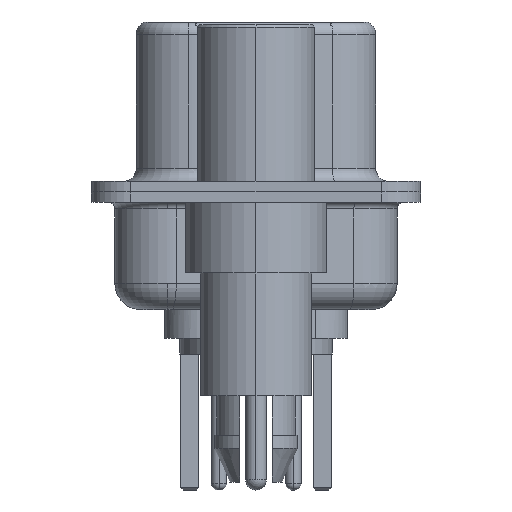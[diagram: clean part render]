
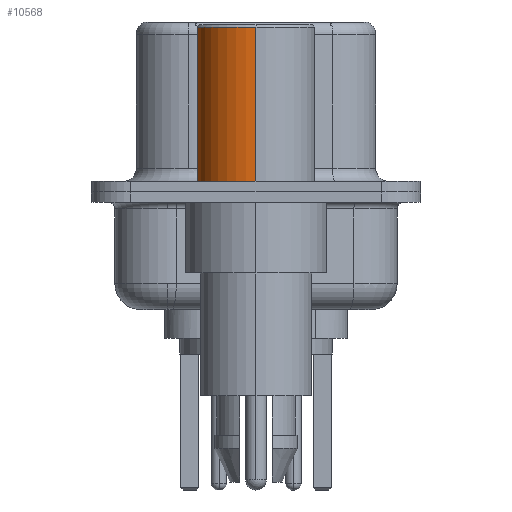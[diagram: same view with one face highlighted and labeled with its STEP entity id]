
A CAD part, left-side view. The second image highlights one B-rep face of the part: STEP entity #10568.
In plain terms, the highlighted cylindrical face has radius 2.25 mm (diameter 4.5 mm), a partial arc.
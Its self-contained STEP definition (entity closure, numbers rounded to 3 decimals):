
#782 = AXIS2_PLACEMENT_3D ( 'NONE', #19846, #8580, #21734 ) ;
#1077 = EDGE_CURVE ( 'NONE', #3015, #3858, #3713, .T. ) ;
#1628 = CYLINDRICAL_SURFACE ( 'NONE', #24458, 2.25 ) ;
#1768 = CARTESIAN_POINT ( 'NONE',  ( 2.25, 0., 0.4 ) ) ;
#3015 = VERTEX_POINT ( 'NONE', #21162 ) ;
#3284 = VERTEX_POINT ( 'NONE', #10674 ) ;
#3713 = CIRCLE ( 'NONE', #12100, 2.25 ) ;
#3714 = VECTOR ( 'NONE', #23561, 1000. ) ;
#3858 = VERTEX_POINT ( 'NONE', #18015 ) ;
#4449 = EDGE_CURVE ( 'NONE', #3284, #3858, #23678, .T. ) ;
#4867 = CARTESIAN_POINT ( 'NONE',  ( 0., 0., 0.581 ) ) ;
#6761 = DIRECTION ( 'NONE',  ( 1., 0., 0. ) ) ;
#6803 = DIRECTION ( 'NONE',  ( 0., 0., 1. ) ) ;
#7287 = FACE_OUTER_BOUND ( 'NONE', #14802, .T. ) ;
#7501 = ORIENTED_EDGE ( 'NONE', *, *, #12702, .F. ) ;
#7556 = CIRCLE ( 'NONE', #782, 2.25 ) ;
#8580 = DIRECTION ( 'NONE',  ( 0., 0., 1. ) ) ;
#8598 = CARTESIAN_POINT ( 'NONE',  ( 0., 0., 6.3 ) ) ;
#8698 = VECTOR ( 'NONE', #17284, 1000. ) ;
#9373 = LINE ( 'NONE', #14204, #3714 ) ;
#10568 = ADVANCED_FACE ( 'NONE', ( #7287 ), #1628, .T. ) ;
#10674 = CARTESIAN_POINT ( 'NONE',  ( -2.25, 0., 0.4 ) ) ;
#10982 = ORIENTED_EDGE ( 'NONE', *, *, #4449, .T. ) ;
#12100 = AXIS2_PLACEMENT_3D ( 'NONE', #8598, #6803, #6761 ) ;
#12702 = EDGE_CURVE ( 'NONE', #19231, #3015, #9373, .T. ) ;
#12870 = ORIENTED_EDGE ( 'NONE', *, *, #1077, .F. ) ;
#13349 = EDGE_CURVE ( 'NONE', #19231, #3284, #7556, .T. ) ;
#13755 = CARTESIAN_POINT ( 'NONE',  ( -2.25, 0., 0.581 ) ) ;
#14204 = CARTESIAN_POINT ( 'NONE',  ( 2.25, 0., 0.581 ) ) ;
#14802 = EDGE_LOOP ( 'NONE', ( #22408, #10982, #12870, #7501 ) ) ;
#16181 = DIRECTION ( 'NONE',  ( 0., 0., 1. ) ) ;
#17284 = DIRECTION ( 'NONE',  ( 0., 0., 1. ) ) ;
#17964 = DIRECTION ( 'NONE',  ( 1., 0., 0. ) ) ;
#18015 = CARTESIAN_POINT ( 'NONE',  ( -2.25, 0., 6.3 ) ) ;
#19231 = VERTEX_POINT ( 'NONE', #1768 ) ;
#19846 = CARTESIAN_POINT ( 'NONE',  ( 0., 0., 0.4 ) ) ;
#21162 = CARTESIAN_POINT ( 'NONE',  ( 2.25, 0., 6.3 ) ) ;
#21734 = DIRECTION ( 'NONE',  ( 1., 0., 0. ) ) ;
#22408 = ORIENTED_EDGE ( 'NONE', *, *, #13349, .T. ) ;
#23561 = DIRECTION ( 'NONE',  ( 0., 0., 1. ) ) ;
#23678 = LINE ( 'NONE', #13755, #8698 ) ;
#24458 = AXIS2_PLACEMENT_3D ( 'NONE', #4867, #16181, #17964 ) ;
